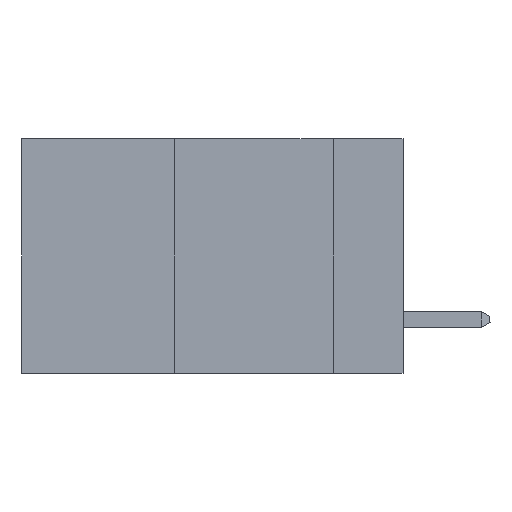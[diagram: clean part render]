
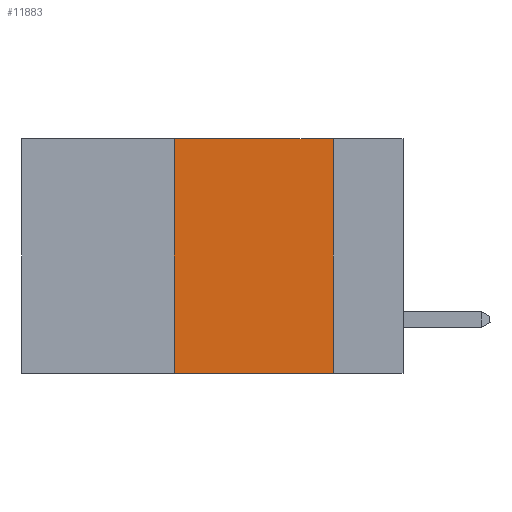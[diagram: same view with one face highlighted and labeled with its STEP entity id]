
A CAD part, left-side view. The second image highlights one B-rep face of the part: STEP entity #11883.
In plain terms, the highlighted planar face has unit normal (-1, 0, 0).
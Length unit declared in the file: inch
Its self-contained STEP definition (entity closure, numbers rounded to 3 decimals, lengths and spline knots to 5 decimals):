
#393 = LINE ( 'NONE', #26324, #22025 ) ;
#1099 = VECTOR ( 'NONE', #1419, 39.37008 ) ;
#1419 = DIRECTION ( 'NONE',  ( 0., 0., -1. ) ) ;
#5297 = CARTESIAN_POINT ( 'NONE',  ( 0., 0.11, 0. ) ) ;
#5527 = CARTESIAN_POINT ( 'NONE',  ( 0., 0.36, -0.37 ) ) ;
#6467 = EDGE_CURVE ( 'NONE', #41931, #15275, #39522, .T. ) ;
#6846 = CARTESIAN_POINT ( 'NONE',  ( 0., 0.6, 0. ) ) ;
#7474 = CARTESIAN_POINT ( 'NONE',  ( 0., 0.11, -0.37 ) ) ;
#10693 = DIRECTION ( 'NONE',  ( 1., 0., 0. ) ) ;
#11001 = EDGE_CURVE ( 'NONE', #42461, #45755, #393, .T. ) ;
#11883 = ADVANCED_FACE ( 'NONE', ( #19580 ), #41075, .F. ) ;
#12526 = LINE ( 'NONE', #5297, #1099 ) ;
#15204 = AXIS2_PLACEMENT_3D ( 'NONE', #6846, #10693, #18084 ) ;
#15275 = VERTEX_POINT ( 'NONE', #7474 ) ;
#18084 = DIRECTION ( 'NONE',  ( 0., 0., -1. ) ) ;
#18197 = VECTOR ( 'NONE', #22201, 39.37008 ) ;
#19342 = DIRECTION ( 'NONE',  ( 0., -1., 0. ) ) ;
#19580 = FACE_OUTER_BOUND ( 'NONE', #34441, .T. ) ;
#22025 = VECTOR ( 'NONE', #37591, 39.37008 ) ;
#22201 = DIRECTION ( 'NONE',  ( 0., 0., 1. ) ) ;
#22580 = ORIENTED_EDGE ( 'NONE', *, *, #31183, .F. ) ;
#25265 = CARTESIAN_POINT ( 'NONE',  ( 0., 0.36, 0. ) ) ;
#26312 = ORIENTED_EDGE ( 'NONE', *, *, #27525, .F. ) ;
#26324 = CARTESIAN_POINT ( 'NONE',  ( 0., 0.6, 0. ) ) ;
#27525 = EDGE_CURVE ( 'NONE', #41931, #42461, #29015, .T. ) ;
#29015 = LINE ( 'NONE', #45232, #18197 ) ;
#31183 = EDGE_CURVE ( 'NONE', #45755, #15275, #12526, .T. ) ;
#34441 = EDGE_LOOP ( 'NONE', ( #22580, #48420, #26312, #45837 ) ) ;
#37591 = DIRECTION ( 'NONE',  ( 0., -1., 0. ) ) ;
#37957 = CARTESIAN_POINT ( 'NONE',  ( 0., 0.6, -0.37 ) ) ;
#39522 = LINE ( 'NONE', #37957, #40101 ) ;
#40101 = VECTOR ( 'NONE', #19342, 39.37008 ) ;
#40940 = CARTESIAN_POINT ( 'NONE',  ( 0., 0.11, 0. ) ) ;
#41075 = PLANE ( 'NONE',  #15204 ) ;
#41931 = VERTEX_POINT ( 'NONE', #5527 ) ;
#42461 = VERTEX_POINT ( 'NONE', #25265 ) ;
#45232 = CARTESIAN_POINT ( 'NONE',  ( 0., 0.36, 0. ) ) ;
#45755 = VERTEX_POINT ( 'NONE', #40940 ) ;
#45837 = ORIENTED_EDGE ( 'NONE', *, *, #6467, .T. ) ;
#48420 = ORIENTED_EDGE ( 'NONE', *, *, #11001, .F. ) ;
